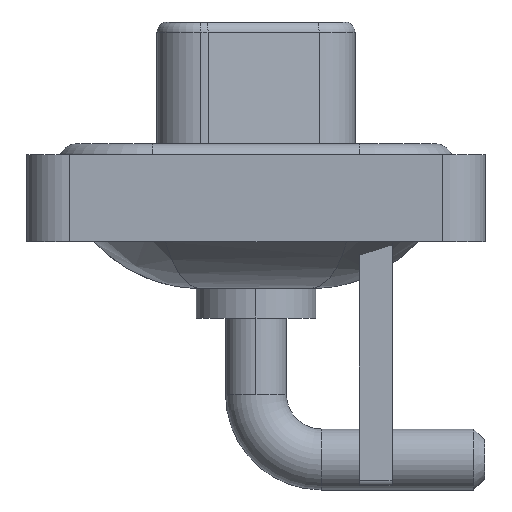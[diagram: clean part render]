
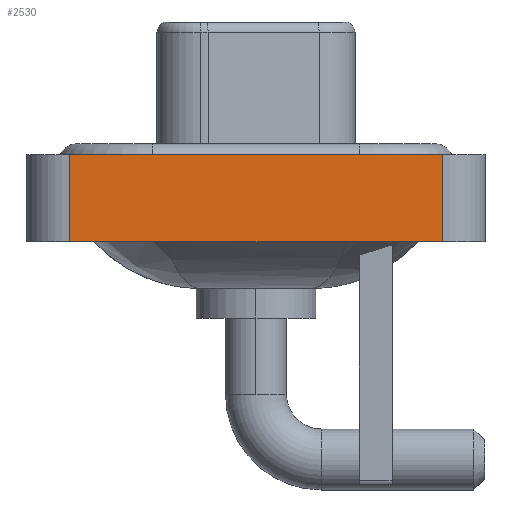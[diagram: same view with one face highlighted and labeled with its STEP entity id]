
A CAD part, left-side view. The second image highlights one B-rep face of the part: STEP entity #2530.
In plain terms, the highlighted planar face has unit normal (-1, 0, 0).
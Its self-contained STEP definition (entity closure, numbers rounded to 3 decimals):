
#204 = PLANE ( 'NONE',  #2964 ) ;
#422 = DIRECTION ( 'NONE',  ( 0., 0., 1. ) ) ;
#1043 = EDGE_CURVE ( 'NONE', #11468, #2524, #2973, .T. ) ;
#1523 = FACE_OUTER_BOUND ( 'NONE', #15079, .T. ) ;
#1613 = CARTESIAN_POINT ( 'NONE',  ( -7.25, 8.55, -3.6 ) ) ;
#2015 = CARTESIAN_POINT ( 'NONE',  ( -7.25, -8.55, 0.4 ) ) ;
#2257 = CARTESIAN_POINT ( 'NONE',  ( -7.25, -8.55, -3.6 ) ) ;
#2274 = LINE ( 'NONE', #16776, #4962 ) ;
#2524 = VERTEX_POINT ( 'NONE', #13619 ) ;
#2530 = ADVANCED_FACE ( 'NONE', ( #1523 ), #204, .T. ) ;
#2964 = AXIS2_PLACEMENT_3D ( 'NONE', #10187, #14623, #17540 ) ;
#2973 = LINE ( 'NONE', #10395, #12710 ) ;
#3756 = ORIENTED_EDGE ( 'NONE', *, *, #4063, .F. ) ;
#4063 = EDGE_CURVE ( 'NONE', #2524, #13048, #2274, .T. ) ;
#4962 = VECTOR ( 'NONE', #15280, 1000. ) ;
#7588 = CARTESIAN_POINT ( 'NONE',  ( -7.25, -8.55, -3.6 ) ) ;
#7662 = LINE ( 'NONE', #10201, #8894 ) ;
#8147 = EDGE_CURVE ( 'NONE', #11468, #15792, #7662, .T. ) ;
#8224 = ORIENTED_EDGE ( 'NONE', *, *, #8147, .T. ) ;
#8641 = VECTOR ( 'NONE', #422, 1000. ) ;
#8724 = ORIENTED_EDGE ( 'NONE', *, *, #13463, .T. ) ;
#8894 = VECTOR ( 'NONE', #16232, 1000. ) ;
#10187 = CARTESIAN_POINT ( 'NONE',  ( -7.25, -8.55, -3.6 ) ) ;
#10201 = CARTESIAN_POINT ( 'NONE',  ( -7.25, -8.55, -3.6 ) ) ;
#10395 = CARTESIAN_POINT ( 'NONE',  ( -7.25, 8.55, -3.6 ) ) ;
#11468 = VERTEX_POINT ( 'NONE', #1613 ) ;
#12078 = ORIENTED_EDGE ( 'NONE', *, *, #1043, .F. ) ;
#12710 = VECTOR ( 'NONE', #17379, 1000. ) ;
#13048 = VERTEX_POINT ( 'NONE', #2015 ) ;
#13463 = EDGE_CURVE ( 'NONE', #15792, #13048, #13520, .T. ) ;
#13520 = LINE ( 'NONE', #7588, #8641 ) ;
#13619 = CARTESIAN_POINT ( 'NONE',  ( -7.25, 8.55, 0.4 ) ) ;
#14623 = DIRECTION ( 'NONE',  ( -1., 0., 0. ) ) ;
#15079 = EDGE_LOOP ( 'NONE', ( #8724, #3756, #12078, #8224 ) ) ;
#15280 = DIRECTION ( 'NONE',  ( 0., -1., 0. ) ) ;
#15792 = VERTEX_POINT ( 'NONE', #2257 ) ;
#16232 = DIRECTION ( 'NONE',  ( 0., -1., 0. ) ) ;
#16776 = CARTESIAN_POINT ( 'NONE',  ( -7.25, -8.55, 0.4 ) ) ;
#17379 = DIRECTION ( 'NONE',  ( 0., 0., 1. ) ) ;
#17540 = DIRECTION ( 'NONE',  ( 0., 0., 1. ) ) ;
